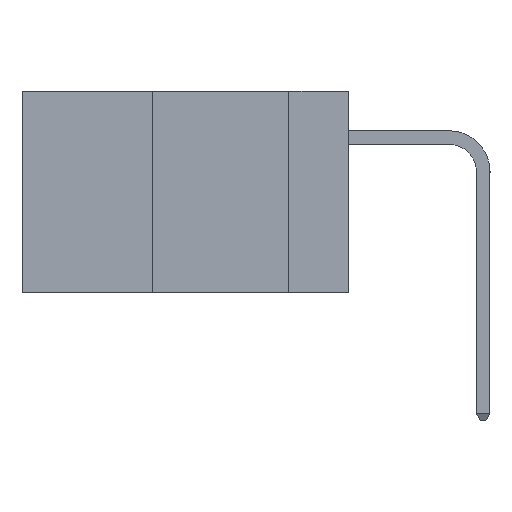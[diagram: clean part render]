
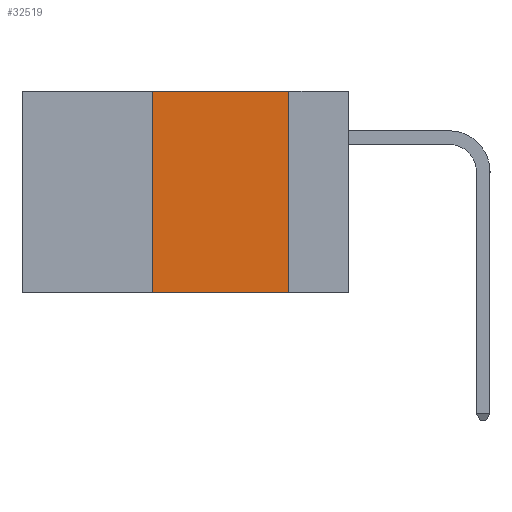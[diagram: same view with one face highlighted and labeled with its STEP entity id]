
A CAD part, left-side view. The second image highlights one B-rep face of the part: STEP entity #32519.
In plain terms, the highlighted planar face has unit normal (-1, 0, 0).
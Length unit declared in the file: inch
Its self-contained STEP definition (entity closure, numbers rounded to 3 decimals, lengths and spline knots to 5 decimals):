
#520 = LINE ( 'NONE', #43159, #45498 ) ;
#2527 = CARTESIAN_POINT ( 'NONE',  ( 0., 0.6, -0.37 ) ) ;
#2890 = VECTOR ( 'NONE', #33296, 39.37008 ) ;
#3837 = ORIENTED_EDGE ( 'NONE', *, *, #33444, .F. ) ;
#4569 = CARTESIAN_POINT ( 'NONE',  ( 0., 0.36, 0. ) ) ;
#5889 = ORIENTED_EDGE ( 'NONE', *, *, #35667, .T. ) ;
#8378 = CARTESIAN_POINT ( 'NONE',  ( 0., 0.11, 0. ) ) ;
#10341 = CARTESIAN_POINT ( 'NONE',  ( 0., 0.36, 0. ) ) ;
#10372 = VERTEX_POINT ( 'NONE', #10341 ) ;
#11774 = VERTEX_POINT ( 'NONE', #45559 ) ;
#13608 = DIRECTION ( 'NONE',  ( 0., -1., 0. ) ) ;
#13694 = AXIS2_PLACEMENT_3D ( 'NONE', #38162, #42270, #41562 ) ;
#13774 = ORIENTED_EDGE ( 'NONE', *, *, #37550, .F. ) ;
#14021 = EDGE_LOOP ( 'NONE', ( #3837, #13774, #28468, #5889 ) ) ;
#15738 = PLANE ( 'NONE',  #13694 ) ;
#18328 = LINE ( 'NONE', #4569, #2890 ) ;
#22579 = VERTEX_POINT ( 'NONE', #37260 ) ;
#25431 = LINE ( 'NONE', #2527, #46158 ) ;
#25919 = EDGE_CURVE ( 'NONE', #31362, #10372, #18328, .T. ) ;
#26717 = LINE ( 'NONE', #8378, #36060 ) ;
#28468 = ORIENTED_EDGE ( 'NONE', *, *, #25919, .F. ) ;
#31362 = VERTEX_POINT ( 'NONE', #46127 ) ;
#32519 = ADVANCED_FACE ( 'NONE', ( #45428 ), #15738, .F. ) ;
#33296 = DIRECTION ( 'NONE',  ( 0., 0., 1. ) ) ;
#33444 = EDGE_CURVE ( 'NONE', #22579, #11774, #26717, .T. ) ;
#35667 = EDGE_CURVE ( 'NONE', #31362, #11774, #25431, .T. ) ;
#36060 = VECTOR ( 'NONE', #37822, 39.37008 ) ;
#36373 = DIRECTION ( 'NONE',  ( 0., -1., 0. ) ) ;
#37260 = CARTESIAN_POINT ( 'NONE',  ( 0., 0.11, 0. ) ) ;
#37550 = EDGE_CURVE ( 'NONE', #10372, #22579, #520, .T. ) ;
#37822 = DIRECTION ( 'NONE',  ( 0., 0., -1. ) ) ;
#38162 = CARTESIAN_POINT ( 'NONE',  ( 0., 0.6, 0. ) ) ;
#41562 = DIRECTION ( 'NONE',  ( 0., 0., -1. ) ) ;
#42270 = DIRECTION ( 'NONE',  ( 1., 0., 0. ) ) ;
#43159 = CARTESIAN_POINT ( 'NONE',  ( 0., 0.6, 0. ) ) ;
#45428 = FACE_OUTER_BOUND ( 'NONE', #14021, .T. ) ;
#45498 = VECTOR ( 'NONE', #36373, 39.37008 ) ;
#45559 = CARTESIAN_POINT ( 'NONE',  ( 0., 0.11, -0.37 ) ) ;
#46127 = CARTESIAN_POINT ( 'NONE',  ( 0., 0.36, -0.37 ) ) ;
#46158 = VECTOR ( 'NONE', #13608, 39.37008 ) ;
